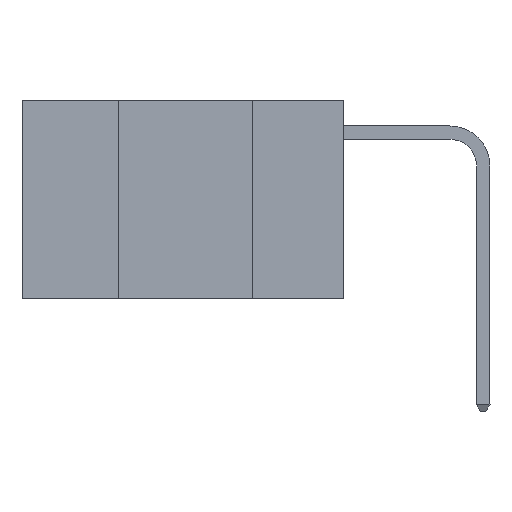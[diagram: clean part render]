
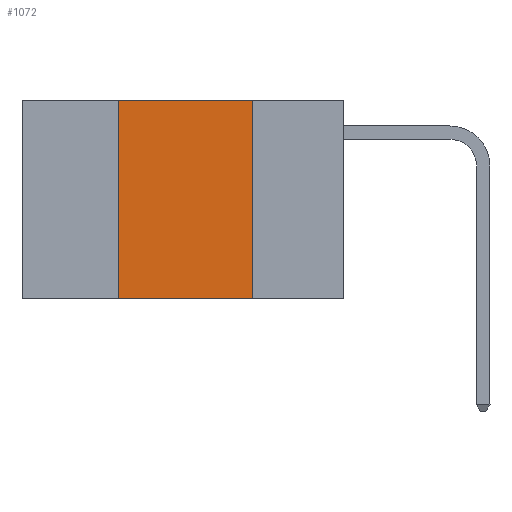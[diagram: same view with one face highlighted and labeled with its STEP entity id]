
A CAD part, left-side view. The second image highlights one B-rep face of the part: STEP entity #1072.
In plain terms, the highlighted planar face has unit normal (-1, 0, 0).
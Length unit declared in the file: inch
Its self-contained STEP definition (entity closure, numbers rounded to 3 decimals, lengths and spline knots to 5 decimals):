
#122 = LINE ( 'NONE', #9849, #2165 ) ;
#530 = EDGE_CURVE ( 'NONE', #7343, #1461, #5778, .T. ) ;
#539 = PLANE ( 'NONE',  #7425 ) ;
#884 = LINE ( 'NONE', #3633, #4625 ) ;
#1072 = ADVANCED_FACE ( 'NONE', ( #1425 ), #539, .F. ) ;
#1175 = ORIENTED_EDGE ( 'NONE', *, *, #1554, .F. ) ;
#1425 = FACE_OUTER_BOUND ( 'NONE', #1436, .T. ) ;
#1436 = EDGE_LOOP ( 'NONE', ( #3954, #1175, #5632, #4261 ) ) ;
#1461 = VERTEX_POINT ( 'NONE', #7881 ) ;
#1554 = EDGE_CURVE ( 'NONE', #2543, #7343, #122, .T. ) ;
#1644 = CARTESIAN_POINT ( 'NONE',  ( 0., 0.17, 0. ) ) ;
#2165 = VECTOR ( 'NONE', #6415, 39.37008 ) ;
#2543 = VERTEX_POINT ( 'NONE', #8905 ) ;
#3633 = CARTESIAN_POINT ( 'NONE',  ( 0., 0.6, -0.37 ) ) ;
#3954 = ORIENTED_EDGE ( 'NONE', *, *, #530, .F. ) ;
#4108 = DIRECTION ( 'NONE',  ( 1., 0., 0. ) ) ;
#4261 = ORIENTED_EDGE ( 'NONE', *, *, #11259, .T. ) ;
#4281 = VECTOR ( 'NONE', #7964, 39.37008 ) ;
#4555 = DIRECTION ( 'NONE',  ( 0., -1., 0. ) ) ;
#4625 = VECTOR ( 'NONE', #4555, 39.37008 ) ;
#5382 = CARTESIAN_POINT ( 'NONE',  ( 0., 0.42, -0.37 ) ) ;
#5632 = ORIENTED_EDGE ( 'NONE', *, *, #7347, .F. ) ;
#5651 = CARTESIAN_POINT ( 'NONE',  ( 0., 0.17, 0. ) ) ;
#5778 = LINE ( 'NONE', #5651, #7027 ) ;
#6199 = CARTESIAN_POINT ( 'NONE',  ( 0., 0.42, 0. ) ) ;
#6415 = DIRECTION ( 'NONE',  ( 0., -1., 0. ) ) ;
#6603 = DIRECTION ( 'NONE',  ( 0., 0., -1. ) ) ;
#7027 = VECTOR ( 'NONE', #6603, 39.37008 ) ;
#7343 = VERTEX_POINT ( 'NONE', #1644 ) ;
#7347 = EDGE_CURVE ( 'NONE', #7407, #2543, #10506, .T. ) ;
#7407 = VERTEX_POINT ( 'NONE', #5382 ) ;
#7425 = AXIS2_PLACEMENT_3D ( 'NONE', #10293, #4108, #9545 ) ;
#7881 = CARTESIAN_POINT ( 'NONE',  ( 0., 0.17, -0.37 ) ) ;
#7964 = DIRECTION ( 'NONE',  ( 0., 0., 1. ) ) ;
#8905 = CARTESIAN_POINT ( 'NONE',  ( 0., 0.42, 0. ) ) ;
#9545 = DIRECTION ( 'NONE',  ( 0., 0., -1. ) ) ;
#9849 = CARTESIAN_POINT ( 'NONE',  ( 0., 0.6, 0. ) ) ;
#10293 = CARTESIAN_POINT ( 'NONE',  ( 0., 0.6, 0. ) ) ;
#10506 = LINE ( 'NONE', #6199, #4281 ) ;
#11259 = EDGE_CURVE ( 'NONE', #7407, #1461, #884, .T. ) ;
